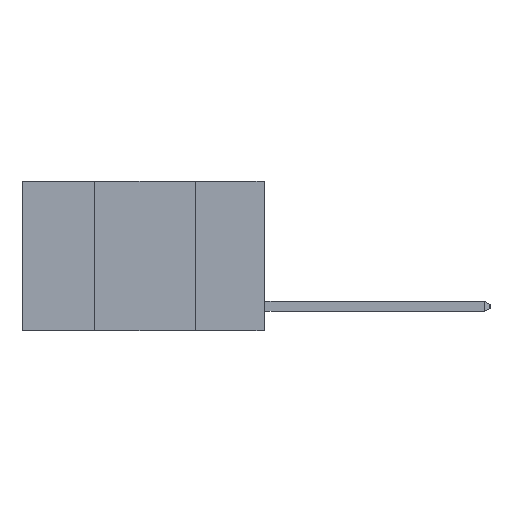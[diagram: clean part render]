
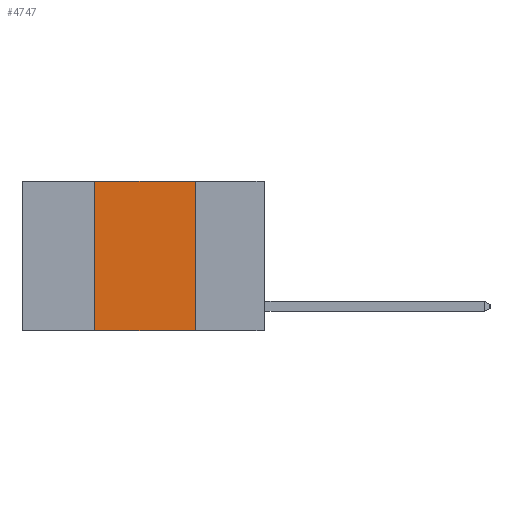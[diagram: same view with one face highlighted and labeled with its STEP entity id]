
A CAD part, left-side view. The second image highlights one B-rep face of the part: STEP entity #4747.
In plain terms, the highlighted planar face has unit normal (-1, 0, 0).
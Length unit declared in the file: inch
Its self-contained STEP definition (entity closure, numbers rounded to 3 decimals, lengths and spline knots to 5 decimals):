
#1492 = VECTOR ( 'NONE', #5164, 39.37008 ) ;
#1664 = ORIENTED_EDGE ( 'NONE', *, *, #5791, .F. ) ;
#1825 = EDGE_CURVE ( 'NONE', #3059, #7843, #5917, .T. ) ;
#1878 = LINE ( 'NONE', #6433, #3674 ) ;
#2253 = CARTESIAN_POINT ( 'NONE',  ( 0., 0.42, 0. ) ) ;
#2368 = CARTESIAN_POINT ( 'NONE',  ( 0., 0.6, 0. ) ) ;
#2647 = DIRECTION ( 'NONE',  ( 0., -1., 0. ) ) ;
#3059 = VERTEX_POINT ( 'NONE', #7884 ) ;
#3147 = DIRECTION ( 'NONE',  ( 1., 0., 0. ) ) ;
#3239 = VERTEX_POINT ( 'NONE', #7641 ) ;
#3504 = LINE ( 'NONE', #7919, #1492 ) ;
#3546 = DIRECTION ( 'NONE',  ( 0., 0., 1. ) ) ;
#3674 = VECTOR ( 'NONE', #8487, 39.37008 ) ;
#3723 = EDGE_CURVE ( 'NONE', #3059, #6440, #5686, .T. ) ;
#4053 = VECTOR ( 'NONE', #2647, 39.37008 ) ;
#4152 = ORIENTED_EDGE ( 'NONE', *, *, #6437, .F. ) ;
#4289 = AXIS2_PLACEMENT_3D ( 'NONE', #2368, #3147, #8055 ) ;
#4307 = EDGE_LOOP ( 'NONE', ( #1664, #4152, #4533, #6228 ) ) ;
#4533 = ORIENTED_EDGE ( 'NONE', *, *, #1825, .F. ) ;
#4747 = ADVANCED_FACE ( 'NONE', ( #6859 ), #6653, .F. ) ;
#4953 = CARTESIAN_POINT ( 'NONE',  ( 0., 0.6, -0.37 ) ) ;
#5164 = DIRECTION ( 'NONE',  ( 0., -1., 0. ) ) ;
#5686 = LINE ( 'NONE', #4953, #4053 ) ;
#5791 = EDGE_CURVE ( 'NONE', #3239, #6440, #1878, .T. ) ;
#5917 = LINE ( 'NONE', #6736, #7598 ) ;
#6228 = ORIENTED_EDGE ( 'NONE', *, *, #3723, .T. ) ;
#6433 = CARTESIAN_POINT ( 'NONE',  ( 0., 0.17, 0. ) ) ;
#6437 = EDGE_CURVE ( 'NONE', #7843, #3239, #3504, .T. ) ;
#6440 = VERTEX_POINT ( 'NONE', #9216 ) ;
#6653 = PLANE ( 'NONE',  #4289 ) ;
#6736 = CARTESIAN_POINT ( 'NONE',  ( 0., 0.42, 0. ) ) ;
#6859 = FACE_OUTER_BOUND ( 'NONE', #4307, .T. ) ;
#7598 = VECTOR ( 'NONE', #3546, 39.37008 ) ;
#7641 = CARTESIAN_POINT ( 'NONE',  ( 0., 0.17, 0. ) ) ;
#7843 = VERTEX_POINT ( 'NONE', #2253 ) ;
#7884 = CARTESIAN_POINT ( 'NONE',  ( 0., 0.42, -0.37 ) ) ;
#7919 = CARTESIAN_POINT ( 'NONE',  ( 0., 0.6, 0. ) ) ;
#8055 = DIRECTION ( 'NONE',  ( 0., 0., -1. ) ) ;
#8487 = DIRECTION ( 'NONE',  ( 0., 0., -1. ) ) ;
#9216 = CARTESIAN_POINT ( 'NONE',  ( 0., 0.17, -0.37 ) ) ;
